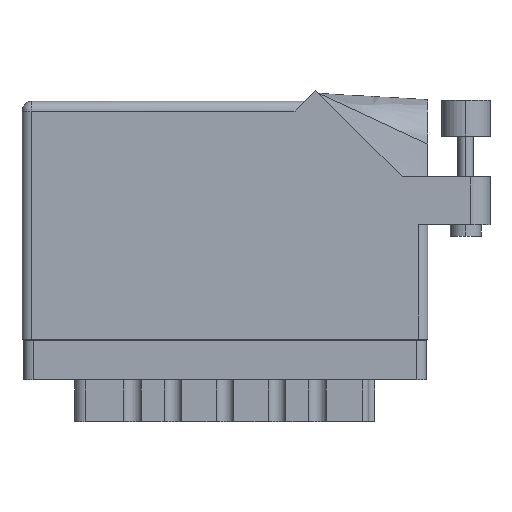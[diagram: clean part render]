
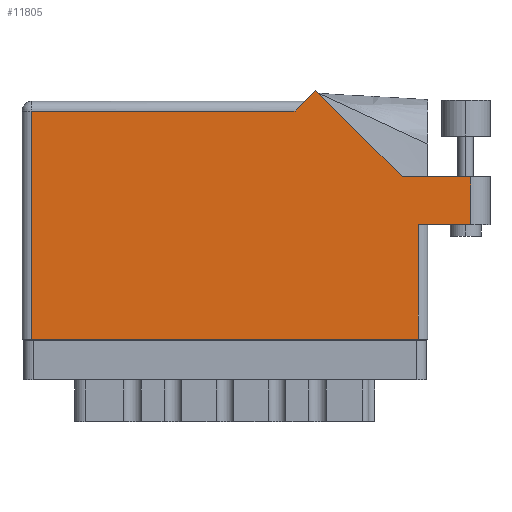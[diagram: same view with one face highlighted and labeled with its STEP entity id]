
A CAD part, front view. The second image highlights one B-rep face of the part: STEP entity #11805.
In plain terms, the highlighted face is planar.
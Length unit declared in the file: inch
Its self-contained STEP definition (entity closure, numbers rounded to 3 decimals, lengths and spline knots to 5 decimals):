
#537 = VECTOR ( 'NONE', #40740, 39.37008 ) ;
#1613 = EDGE_CURVE ( 'NONE', #15794, #4809, #30218, .T. ) ;
#3289 = ORIENTED_EDGE ( 'NONE', *, *, #37778, .T. ) ;
#3546 = VERTEX_POINT ( 'NONE', #36716 ) ;
#3965 = DIRECTION ( 'NONE',  ( 0., -1., 0. ) ) ;
#4767 = VECTOR ( 'NONE', #37490, 39.37008 ) ;
#4809 = VERTEX_POINT ( 'NONE', #12449 ) ;
#5377 = VECTOR ( 'NONE', #48511, 39.37008 ) ;
#7423 = EDGE_CURVE ( 'NONE', #26500, #15794, #48266, .T. ) ;
#8801 = ORIENTED_EDGE ( 'NONE', *, *, #7423, .T. ) ;
#9290 = DIRECTION ( 'NONE',  ( 1., 0., 0. ) ) ;
#10141 = DIRECTION ( 'NONE',  ( -1., 0., 0. ) ) ;
#10690 = LINE ( 'NONE', #29002, #537 ) ;
#11805 = ADVANCED_FACE ( 'NONE', ( #12473 ), #13668, .F. ) ;
#12117 = CARTESIAN_POINT ( 'NONE',  ( 0.062, 0., 0. ) ) ;
#12449 = CARTESIAN_POINT ( 'NONE',  ( 2.55, 0., 0. ) ) ;
#12473 = FACE_OUTER_BOUND ( 'NONE', #31894, .T. ) ;
#13090 = VERTEX_POINT ( 'NONE', #37582 ) ;
#13668 = PLANE ( 'NONE',  #24793 ) ;
#13857 = VECTOR ( 'NONE', #31495, 39.37008 ) ;
#15609 = CARTESIAN_POINT ( 'NONE',  ( 1.88971, 1.60071, 0. ) ) ;
#15794 = VERTEX_POINT ( 'NONE', #35591 ) ;
#15903 = CARTESIAN_POINT ( 'NONE',  ( 2.55, 0.737, 0. ) ) ;
#16106 = LINE ( 'NONE', #26592, #4767 ) ;
#17191 = DIRECTION ( 'NONE',  ( 0., 1., 0. ) ) ;
#18391 = ORIENTED_EDGE ( 'NONE', *, *, #41963, .T. ) ;
#19258 = LINE ( 'NONE', #24467, #40212 ) ;
#19384 = CARTESIAN_POINT ( 'NONE',  ( 0.062, 1.468, 0. ) ) ;
#20393 = LINE ( 'NONE', #42750, #13857 ) ;
#20424 = VERTEX_POINT ( 'NONE', #15903 ) ;
#20886 = LINE ( 'NONE', #45344, #5377 ) ;
#21451 = ORIENTED_EDGE ( 'NONE', *, *, #1613, .T. ) ;
#21976 = DIRECTION ( 'NONE',  ( 0., 0., -1. ) ) ;
#23592 = VECTOR ( 'NONE', #24397, 39.37008 ) ;
#24397 = DIRECTION ( 'NONE',  ( 0., 1., 0. ) ) ;
#24467 = CARTESIAN_POINT ( 'NONE',  ( 2.612, 0.737, 0. ) ) ;
#24793 = AXIS2_PLACEMENT_3D ( 'NONE', #29154, #21976, #10141 ) ;
#25419 = ORIENTED_EDGE ( 'NONE', *, *, #29909, .T. ) ;
#25713 = ORIENTED_EDGE ( 'NONE', *, *, #43509, .T. ) ;
#25798 = VERTEX_POINT ( 'NONE', #15609 ) ;
#26500 = VERTEX_POINT ( 'NONE', #19384 ) ;
#26592 = CARTESIAN_POINT ( 'NONE',  ( 3.012, 1.044, 0. ) ) ;
#27158 = LINE ( 'NONE', #31928, #23592 ) ;
#27176 = VERTEX_POINT ( 'NONE', #28114 ) ;
#27676 = VERTEX_POINT ( 'NONE', #43617 ) ;
#28114 = CARTESIAN_POINT ( 'NONE',  ( 2.44642, 1.044, 0. ) ) ;
#29002 = CARTESIAN_POINT ( 'NONE',  ( 0., 1.468, 0. ) ) ;
#29154 = CARTESIAN_POINT ( 'NONE',  ( 0., 1.53, 0. ) ) ;
#29909 = EDGE_CURVE ( 'NONE', #4809, #20424, #46971, .T. ) ;
#30055 = CARTESIAN_POINT ( 'NONE',  ( 0., 0., 0. ) ) ;
#30218 = LINE ( 'NONE', #30055, #49413 ) ;
#30897 = EDGE_CURVE ( 'NONE', #20424, #3546, #19258, .T. ) ;
#31495 = DIRECTION ( 'NONE',  ( -0.707, 0.707, 0. ) ) ;
#31894 = EDGE_LOOP ( 'NONE', ( #49201, #3289, #37925, #18391, #25713, #37047, #8801, #21451, #25419 ) ) ;
#31928 = CARTESIAN_POINT ( 'NONE',  ( 2.887, 1.044, 0. ) ) ;
#35591 = CARTESIAN_POINT ( 'NONE',  ( 0.062, 0., 0. ) ) ;
#35699 = CARTESIAN_POINT ( 'NONE',  ( 2.55, 0.737, 0. ) ) ;
#36716 = CARTESIAN_POINT ( 'NONE',  ( 2.887, 0.737, 0. ) ) ;
#37047 = ORIENTED_EDGE ( 'NONE', *, *, #43969, .T. ) ;
#37490 = DIRECTION ( 'NONE',  ( -1., 0., 0. ) ) ;
#37582 = CARTESIAN_POINT ( 'NONE',  ( 2.887, 1.044, 0. ) ) ;
#37778 = EDGE_CURVE ( 'NONE', #3546, #13090, #27158, .T. ) ;
#37925 = ORIENTED_EDGE ( 'NONE', *, *, #42974, .T. ) ;
#40212 = VECTOR ( 'NONE', #9290, 39.37008 ) ;
#40740 = DIRECTION ( 'NONE',  ( -1., 0., 0. ) ) ;
#41031 = VECTOR ( 'NONE', #3965, 39.37008 ) ;
#41639 = DIRECTION ( 'NONE',  ( 1., 0., 0. ) ) ;
#41963 = EDGE_CURVE ( 'NONE', #27176, #25798, #20393, .T. ) ;
#42750 = CARTESIAN_POINT ( 'NONE',  ( 2.44642, 1.044, 0. ) ) ;
#42974 = EDGE_CURVE ( 'NONE', #13090, #27176, #16106, .T. ) ;
#43509 = EDGE_CURVE ( 'NONE', #25798, #27676, #20886, .T. ) ;
#43617 = CARTESIAN_POINT ( 'NONE',  ( 1.757, 1.468, 0. ) ) ;
#43969 = EDGE_CURVE ( 'NONE', #27676, #26500, #10690, .T. ) ;
#45344 = CARTESIAN_POINT ( 'NONE',  ( 1.819, 1.53, 0. ) ) ;
#46971 = LINE ( 'NONE', #35699, #49354 ) ;
#48266 = LINE ( 'NONE', #12117, #41031 ) ;
#48511 = DIRECTION ( 'NONE',  ( -0.707, -0.707, 0. ) ) ;
#49201 = ORIENTED_EDGE ( 'NONE', *, *, #30897, .T. ) ;
#49354 = VECTOR ( 'NONE', #17191, 39.37008 ) ;
#49413 = VECTOR ( 'NONE', #41639, 39.37008 ) ;
